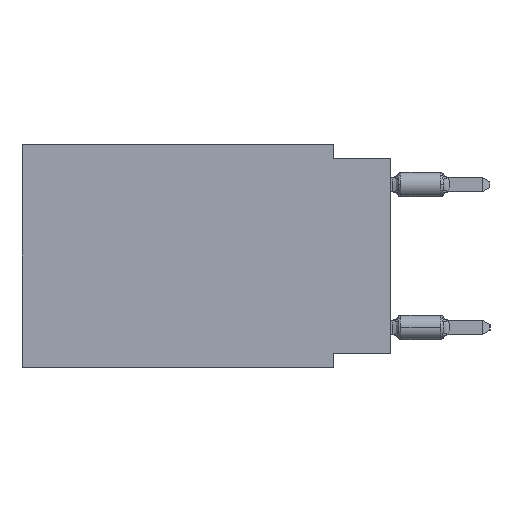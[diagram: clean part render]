
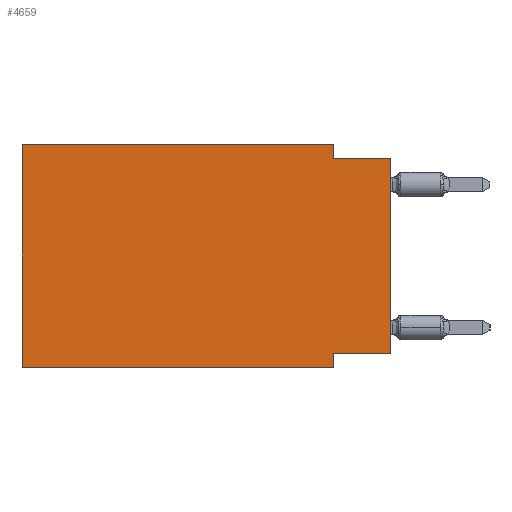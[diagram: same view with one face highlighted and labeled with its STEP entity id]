
A CAD part, left-side view. The second image highlights one B-rep face of the part: STEP entity #4659.
In plain terms, the highlighted planar face has unit normal (-1, 0, 0).
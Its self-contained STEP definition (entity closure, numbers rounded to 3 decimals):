
#259 = VECTOR ( 'NONE', #38232, 1000. ) ;
#545 = CARTESIAN_POINT ( 'NONE',  ( 0., 2.54, -0.635 ) ) ;
#1627 = EDGE_LOOP ( 'NONE', ( #59601, #42671, #8893, #50349, #56879, #31963, #10120, #25349 ) ) ;
#2539 = VERTEX_POINT ( 'NONE', #7969 ) ;
#3409 = DIRECTION ( 'NONE',  ( 0., -1., 0. ) ) ;
#3611 = LINE ( 'NONE', #16520, #49880 ) ;
#4174 = LINE ( 'NONE', #41602, #5054 ) ;
#4659 = ADVANCED_FACE ( 'NONE', ( #29188 ), #29798, .F. ) ;
#4770 = DIRECTION ( 'NONE',  ( 0., 0., 1. ) ) ;
#5054 = VECTOR ( 'NONE', #4770, 1000. ) ;
#6712 = LINE ( 'NONE', #30331, #49577 ) ;
#7291 = EDGE_CURVE ( 'NONE', #44202, #47910, #52271, .T. ) ;
#7964 = CARTESIAN_POINT ( 'NONE',  ( 0., 2.54, -9.271 ) ) ;
#7969 = CARTESIAN_POINT ( 'NONE',  ( 0., 2.54, 0. ) ) ;
#8893 = ORIENTED_EDGE ( 'NONE', *, *, #33710, .F. ) ;
#9036 = EDGE_CURVE ( 'NONE', #35158, #54470, #35613, .T. ) ;
#9645 = EDGE_CURVE ( 'NONE', #44202, #54470, #57127, .T. ) ;
#10120 = ORIENTED_EDGE ( 'NONE', *, *, #19766, .F. ) ;
#13323 = CARTESIAN_POINT ( 'NONE',  ( 0., 0., -0.635 ) ) ;
#14833 = DIRECTION ( 'NONE',  ( 0., 1., 0. ) ) ;
#15142 = CARTESIAN_POINT ( 'NONE',  ( 0., 0., -9.271 ) ) ;
#15244 = LINE ( 'NONE', #30801, #259 ) ;
#16520 = CARTESIAN_POINT ( 'NONE',  ( 0., 2.54, -9.906 ) ) ;
#16922 = CARTESIAN_POINT ( 'NONE',  ( 0., 0., -0.635 ) ) ;
#19716 = VECTOR ( 'NONE', #45669, 1000. ) ;
#19766 = EDGE_CURVE ( 'NONE', #47910, #34174, #3611, .T. ) ;
#22077 = CARTESIAN_POINT ( 'NONE',  ( 0., 16.383, 0. ) ) ;
#22666 = EDGE_CURVE ( 'NONE', #23154, #2539, #35853, .T. ) ;
#23154 = VERTEX_POINT ( 'NONE', #53598 ) ;
#23192 = EDGE_CURVE ( 'NONE', #24120, #23154, #4174, .T. ) ;
#24120 = VERTEX_POINT ( 'NONE', #39471 ) ;
#24291 = DIRECTION ( 'NONE',  ( 1., 0., 0. ) ) ;
#24900 = DIRECTION ( 'NONE',  ( 0., 0., -1. ) ) ;
#25349 = ORIENTED_EDGE ( 'NONE', *, *, #7291, .F. ) ;
#29188 = FACE_OUTER_BOUND ( 'NONE', #1627, .T. ) ;
#29798 = PLANE ( 'NONE',  #34356 ) ;
#30179 = CARTESIAN_POINT ( 'NONE',  ( 0., 2.54, -9.906 ) ) ;
#30196 = EDGE_CURVE ( 'NONE', #24120, #34174, #15244, .T. ) ;
#30331 = CARTESIAN_POINT ( 'NONE',  ( 0., 2.54, 0. ) ) ;
#30801 = CARTESIAN_POINT ( 'NONE',  ( 0., 16.383, -9.906 ) ) ;
#31963 = ORIENTED_EDGE ( 'NONE', *, *, #30196, .T. ) ;
#33710 = EDGE_CURVE ( 'NONE', #2539, #35158, #6712, .T. ) ;
#34174 = VERTEX_POINT ( 'NONE', #30179 ) ;
#34356 = AXIS2_PLACEMENT_3D ( 'NONE', #38676, #24291, #24900 ) ;
#35158 = VERTEX_POINT ( 'NONE', #545 ) ;
#35537 = DIRECTION ( 'NONE',  ( 0., 0., -1. ) ) ;
#35613 = LINE ( 'NONE', #16922, #38771 ) ;
#35853 = LINE ( 'NONE', #22077, #19716 ) ;
#38089 = DIRECTION ( 'NONE',  ( 0., 0., 1. ) ) ;
#38232 = DIRECTION ( 'NONE',  ( 0., -1., 0. ) ) ;
#38676 = CARTESIAN_POINT ( 'NONE',  ( 0., 16.383, 0. ) ) ;
#38771 = VECTOR ( 'NONE', #3409, 1000. ) ;
#39471 = CARTESIAN_POINT ( 'NONE',  ( 0., 16.383, -9.906 ) ) ;
#41602 = CARTESIAN_POINT ( 'NONE',  ( 0., 16.383, 0. ) ) ;
#42411 = VECTOR ( 'NONE', #14833, 1000. ) ;
#42671 = ORIENTED_EDGE ( 'NONE', *, *, #9036, .F. ) ;
#44202 = VERTEX_POINT ( 'NONE', #55553 ) ;
#45669 = DIRECTION ( 'NONE',  ( 0., -1., 0. ) ) ;
#45924 = DIRECTION ( 'NONE',  ( 0., 0., -1. ) ) ;
#47910 = VERTEX_POINT ( 'NONE', #7964 ) ;
#49577 = VECTOR ( 'NONE', #35537, 1000. ) ;
#49880 = VECTOR ( 'NONE', #45924, 1000. ) ;
#50349 = ORIENTED_EDGE ( 'NONE', *, *, #22666, .F. ) ;
#52271 = LINE ( 'NONE', #15142, #42411 ) ;
#52538 = CARTESIAN_POINT ( 'NONE',  ( 0., 0., 0. ) ) ;
#53598 = CARTESIAN_POINT ( 'NONE',  ( 0., 16.383, 0. ) ) ;
#54470 = VERTEX_POINT ( 'NONE', #13323 ) ;
#55553 = CARTESIAN_POINT ( 'NONE',  ( 0., 0., -9.271 ) ) ;
#56879 = ORIENTED_EDGE ( 'NONE', *, *, #23192, .F. ) ;
#57127 = LINE ( 'NONE', #52538, #60386 ) ;
#59601 = ORIENTED_EDGE ( 'NONE', *, *, #9645, .T. ) ;
#60386 = VECTOR ( 'NONE', #38089, 1000. ) ;
